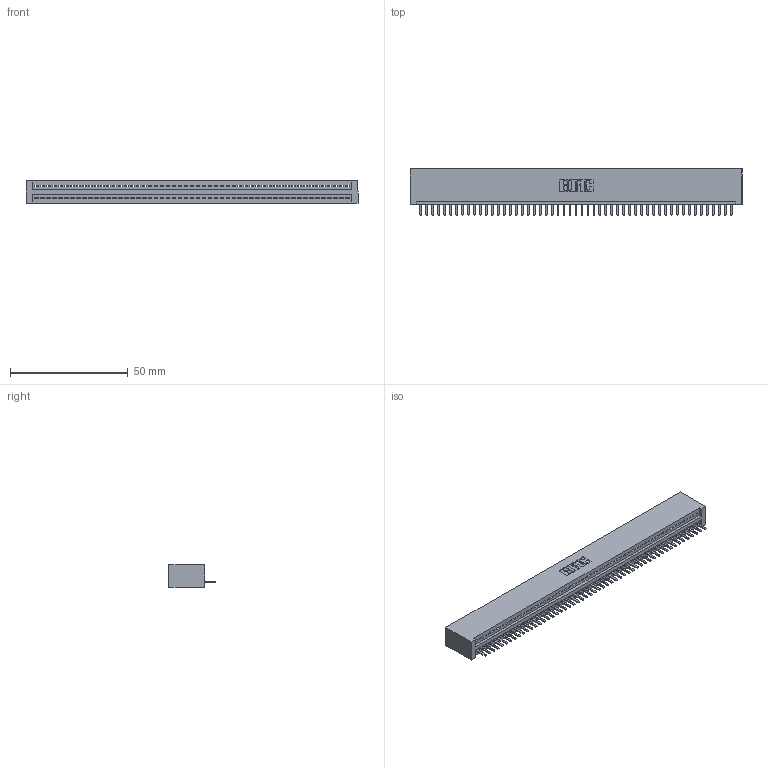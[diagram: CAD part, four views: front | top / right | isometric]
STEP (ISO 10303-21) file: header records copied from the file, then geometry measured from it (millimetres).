
FILE_DESCRIPTION (( 'STEP AP203' ), '1' );
FILE_NAME ('395-053-520-101.STEP', '2019-10-23T13:45:17', ( '' ), ( '' ), 'SwSTEP 2.0', 'SolidWorks 2016', '' );
FILE_SCHEMA (( 'CONFIG_CONTROL_DESIGN' ));
Length unit declared in the file: inch
Products named in the file (3): 395-053-520-101; 345 Part_No Mounting Lugs; 345-292-001_345-293-120
Assembly tree (54 placements, depth 2):
  395-053-520-101
    345 Part_No Mounting Lugs
    345-292-001_345-293-120  x53
Bounding box: 141.22 x 19.68 x 9.4 mm (x, y, z)
Volume: 13935.6 mm3; surface area: 18360.1 mm2
Topology: 54 solids, 54 shells, 3404 faces, 10069 edges, 6570 vertices
Faces by surface type: plane 2302, cylinder 1102
Entity records: 38245 total; most frequent: CARTESIAN_POINT 6643, ORIENTED_EDGE 6618, DIRECTION 5767, EDGE_CURVE 3309, VECTOR 2969, LINE 2969, VERTEX_POINT 2202, AXIS2_PLACEMENT_3D 1399
